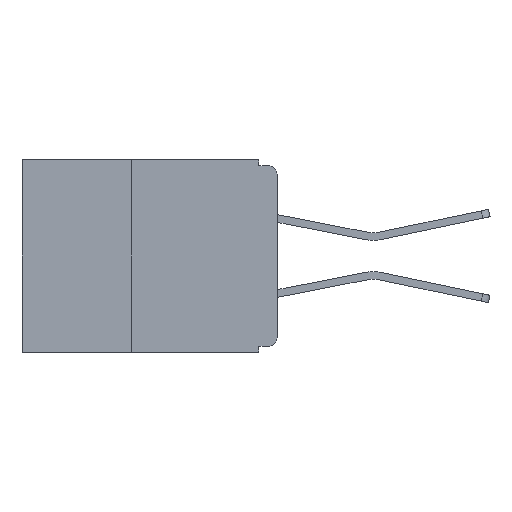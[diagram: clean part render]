
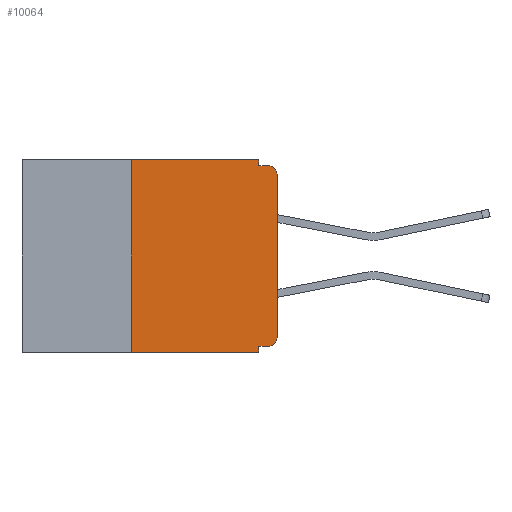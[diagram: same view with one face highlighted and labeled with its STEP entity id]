
A CAD part, left-side view. The second image highlights one B-rep face of the part: STEP entity #10064.
In plain terms, the highlighted planar face has unit normal (-1, 0, 0).
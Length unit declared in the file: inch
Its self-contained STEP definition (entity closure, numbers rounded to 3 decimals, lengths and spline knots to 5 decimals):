
#763 = ORIENTED_EDGE ( 'NONE', *, *, #7401, .T. ) ;
#848 = CIRCLE ( 'NONE', #3209, 0.015 ) ;
#1877 = ORIENTED_EDGE ( 'NONE', *, *, #22853, .T. ) ;
#1931 = LINE ( 'NONE', #11276, #7524 ) ;
#2071 = CARTESIAN_POINT ( 'NONE',  ( 0., 0.437, 0. ) ) ;
#2272 = ORIENTED_EDGE ( 'NONE', *, *, #2604, .T. ) ;
#2604 = EDGE_CURVE ( 'NONE', #3960, #7996, #22696, .T. ) ;
#3015 = VERTEX_POINT ( 'NONE', #9205 ) ;
#3209 = AXIS2_PLACEMENT_3D ( 'NONE', #27875, #13642, #30316 ) ;
#3340 = CARTESIAN_POINT ( 'NONE',  ( 0., 0.25, -0.33 ) ) ;
#3756 = ORIENTED_EDGE ( 'NONE', *, *, #15362, .F. ) ;
#3960 = VERTEX_POINT ( 'NONE', #25435 ) ;
#4977 = VECTOR ( 'NONE', #20024, 39.37008 ) ;
#5424 = DIRECTION ( 'NONE',  ( 0., 1., 0. ) ) ;
#7380 = VECTOR ( 'NONE', #29457, 39.37008 ) ;
#7401 = EDGE_CURVE ( 'NONE', #24458, #17908, #27505, .T. ) ;
#7524 = VECTOR ( 'NONE', #13695, 39.37008 ) ;
#7613 = LINE ( 'NONE', #10299, #11727 ) ;
#7766 = VERTEX_POINT ( 'NONE', #26650 ) ;
#7809 = CARTESIAN_POINT ( 'NONE',  ( 0., 0.031, -0.33 ) ) ;
#7996 = VERTEX_POINT ( 'NONE', #22678 ) ;
#8137 = CARTESIAN_POINT ( 'NONE',  ( 0., 0.031, -0.33 ) ) ;
#9205 = CARTESIAN_POINT ( 'NONE',  ( 0., 0.015, -0.32 ) ) ;
#9621 = EDGE_CURVE ( 'NONE', #28560, #17908, #13990, .T. ) ;
#9824 = DIRECTION ( 'NONE',  ( -1., 0., 0. ) ) ;
#10064 = ADVANCED_FACE ( 'NONE', ( #20292 ), #28294, .F. ) ;
#10216 = DIRECTION ( 'NONE',  ( 0., 0., -1. ) ) ;
#10299 = CARTESIAN_POINT ( 'NONE',  ( 0., 0.031, 0. ) ) ;
#10855 = VERTEX_POINT ( 'NONE', #25098 ) ;
#10862 = ORIENTED_EDGE ( 'NONE', *, *, #21058, .F. ) ;
#11276 = CARTESIAN_POINT ( 'NONE',  ( 0., 0.437, 0. ) ) ;
#11285 = LINE ( 'NONE', #3340, #4977 ) ;
#11719 = CARTESIAN_POINT ( 'NONE',  ( 0., 0.031, -0.01 ) ) ;
#11727 = VECTOR ( 'NONE', #22172, 39.37008 ) ;
#12379 = CARTESIAN_POINT ( 'NONE',  ( 0., 0.25, 0. ) ) ;
#13257 = DIRECTION ( 'NONE',  ( 0., 0., 1. ) ) ;
#13362 = CARTESIAN_POINT ( 'NONE',  ( 0., 0.031, -0.32 ) ) ;
#13642 = DIRECTION ( 'NONE',  ( -1., 0., 0. ) ) ;
#13695 = DIRECTION ( 'NONE',  ( 0., -1., 0. ) ) ;
#13990 = LINE ( 'NONE', #7809, #30765 ) ;
#14070 = DIRECTION ( 'NONE',  ( 1., 0., 0. ) ) ;
#14859 = CARTESIAN_POINT ( 'NONE',  ( 0., 0., 0. ) ) ;
#15362 = EDGE_CURVE ( 'NONE', #3015, #28560, #23697, .T. ) ;
#15762 = VERTEX_POINT ( 'NONE', #12379 ) ;
#16372 = VECTOR ( 'NONE', #27599, 39.37008 ) ;
#16404 = VECTOR ( 'NONE', #13257, 39.37008 ) ;
#16840 = EDGE_CURVE ( 'NONE', #7996, #7766, #848, .T. ) ;
#17204 = ORIENTED_EDGE ( 'NONE', *, *, #16840, .T. ) ;
#17260 = ORIENTED_EDGE ( 'NONE', *, *, #21692, .F. ) ;
#17908 = VERTEX_POINT ( 'NONE', #8137 ) ;
#18176 = CARTESIAN_POINT ( 'NONE',  ( 0., 0.437, -0.33 ) ) ;
#18935 = AXIS2_PLACEMENT_3D ( 'NONE', #24075, #9824, #26477 ) ;
#19894 = CARTESIAN_POINT ( 'NONE',  ( 0., 0., -0.32 ) ) ;
#20024 = DIRECTION ( 'NONE',  ( 0., 0., 1. ) ) ;
#20292 = FACE_OUTER_BOUND ( 'NONE', #24430, .T. ) ;
#21058 = EDGE_CURVE ( 'NONE', #10855, #27169, #7613, .T. ) ;
#21284 = CIRCLE ( 'NONE', #18935, 0.015 ) ;
#21561 = LINE ( 'NONE', #24633, #7380 ) ;
#21692 = EDGE_CURVE ( 'NONE', #24458, #15762, #11285, .T. ) ;
#22172 = DIRECTION ( 'NONE',  ( 0., 0., -1. ) ) ;
#22678 = CARTESIAN_POINT ( 'NONE',  ( 0., 0., -0.025 ) ) ;
#22696 = LINE ( 'NONE', #14859, #16404 ) ;
#22853 = EDGE_CURVE ( 'NONE', #3015, #3960, #21284, .T. ) ;
#23141 = ORIENTED_EDGE ( 'NONE', *, *, #30921, .F. ) ;
#23697 = LINE ( 'NONE', #19894, #30074 ) ;
#24075 = CARTESIAN_POINT ( 'NONE',  ( 0., 0.015, -0.305 ) ) ;
#24430 = EDGE_LOOP ( 'NONE', ( #2272, #17204, #23141, #10862, #28774, #17260, #763, #28356, #3756, #1877 ) ) ;
#24458 = VERTEX_POINT ( 'NONE', #28056 ) ;
#24633 = CARTESIAN_POINT ( 'NONE',  ( 0., 0., -0.01 ) ) ;
#25098 = CARTESIAN_POINT ( 'NONE',  ( 0., 0.031, 0. ) ) ;
#25435 = CARTESIAN_POINT ( 'NONE',  ( 0., 0., -0.305 ) ) ;
#26477 = DIRECTION ( 'NONE',  ( 0., 0., -1. ) ) ;
#26650 = CARTESIAN_POINT ( 'NONE',  ( 0., 0.015, -0.01 ) ) ;
#27169 = VERTEX_POINT ( 'NONE', #11719 ) ;
#27505 = LINE ( 'NONE', #18176, #16372 ) ;
#27599 = DIRECTION ( 'NONE',  ( 0., -1., 0. ) ) ;
#27875 = CARTESIAN_POINT ( 'NONE',  ( 0., 0.015, -0.025 ) ) ;
#28011 = EDGE_CURVE ( 'NONE', #15762, #10855, #1931, .T. ) ;
#28056 = CARTESIAN_POINT ( 'NONE',  ( 0., 0.25, -0.33 ) ) ;
#28081 = AXIS2_PLACEMENT_3D ( 'NONE', #2071, #14070, #30745 ) ;
#28294 = PLANE ( 'NONE',  #28081 ) ;
#28356 = ORIENTED_EDGE ( 'NONE', *, *, #9621, .F. ) ;
#28560 = VERTEX_POINT ( 'NONE', #13362 ) ;
#28774 = ORIENTED_EDGE ( 'NONE', *, *, #28011, .F. ) ;
#29457 = DIRECTION ( 'NONE',  ( 0., -1., 0. ) ) ;
#30074 = VECTOR ( 'NONE', #5424, 39.37008 ) ;
#30316 = DIRECTION ( 'NONE',  ( 0., 0., -1. ) ) ;
#30745 = DIRECTION ( 'NONE',  ( 0., 0., -1. ) ) ;
#30765 = VECTOR ( 'NONE', #10216, 39.37008 ) ;
#30921 = EDGE_CURVE ( 'NONE', #27169, #7766, #21561, .T. ) ;
